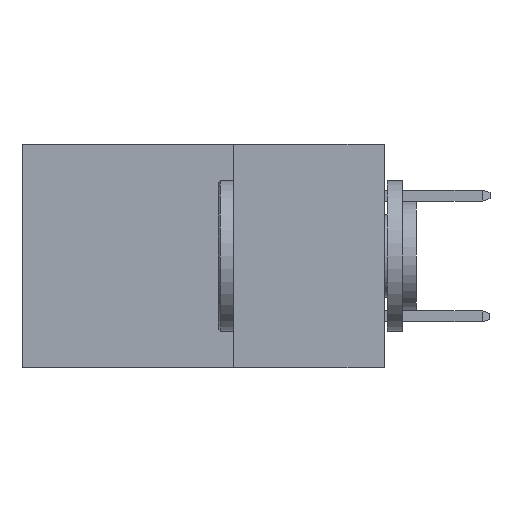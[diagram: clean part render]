
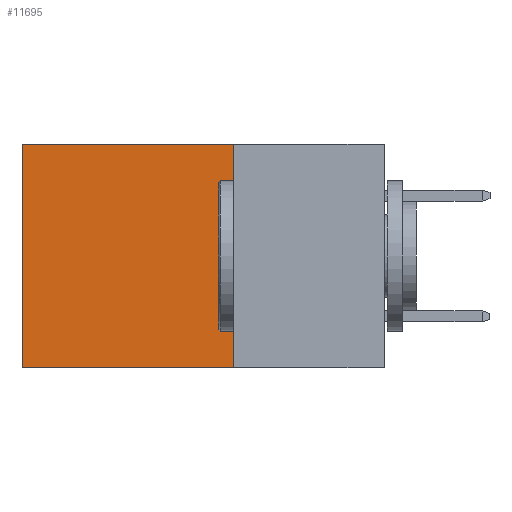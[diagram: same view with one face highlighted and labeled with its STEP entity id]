
A CAD part, left-side view. The second image highlights one B-rep face of the part: STEP entity #11695.
In plain terms, the highlighted planar face has unit normal (-1, 0, 0).
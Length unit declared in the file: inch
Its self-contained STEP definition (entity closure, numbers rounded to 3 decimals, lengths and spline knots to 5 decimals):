
#1762 = CARTESIAN_POINT ( 'NONE',  ( 0.298, 0.25, -0.37 ) ) ;
#3369 = AXIS2_PLACEMENT_3D ( 'NONE', #10174, #11344, #4335 ) ;
#3445 = LINE ( 'NONE', #13287, #9369 ) ;
#3631 = VERTEX_POINT ( 'NONE', #9866 ) ;
#4335 = DIRECTION ( 'NONE',  ( 0., 0., -1. ) ) ;
#4357 = CARTESIAN_POINT ( 'NONE',  ( 0.298, 0.25, 0. ) ) ;
#4647 = CARTESIAN_POINT ( 'NONE',  ( 0.298, 0.25, 0. ) ) ;
#4777 = CARTESIAN_POINT ( 'NONE',  ( 0.298, 0.25, -0.37 ) ) ;
#4915 = VERTEX_POINT ( 'NONE', #11802 ) ;
#5357 = CARTESIAN_POINT ( 'NONE',  ( 0.298, 0.6, 0. ) ) ;
#5767 = EDGE_CURVE ( 'NONE', #6051, #3631, #13843, .T. ) ;
#6051 = VERTEX_POINT ( 'NONE', #4647 ) ;
#7215 = ORIENTED_EDGE ( 'NONE', *, *, #11619, .T. ) ;
#7419 = ORIENTED_EDGE ( 'NONE', *, *, #12192, .F. ) ;
#7812 = PLANE ( 'NONE',  #3369 ) ;
#7878 = VECTOR ( 'NONE', #8910, 39.37008 ) ;
#8002 = VERTEX_POINT ( 'NONE', #1762 ) ;
#8353 = VECTOR ( 'NONE', #15155, 39.37008 ) ;
#8500 = ORIENTED_EDGE ( 'NONE', *, *, #9016, .F. ) ;
#8611 = EDGE_LOOP ( 'NONE', ( #7215, #8500, #7419, #14682 ) ) ;
#8910 = DIRECTION ( 'NONE',  ( 0., 0., -1. ) ) ;
#9016 = EDGE_CURVE ( 'NONE', #8002, #4915, #11465, .T. ) ;
#9369 = VECTOR ( 'NONE', #11075, 39.37008 ) ;
#9866 = CARTESIAN_POINT ( 'NONE',  ( 0.298, 0.6, 0. ) ) ;
#10174 = CARTESIAN_POINT ( 'NONE',  ( 0.298, 0.25, 0. ) ) ;
#10827 = VECTOR ( 'NONE', #12020, 39.37008 ) ;
#11075 = DIRECTION ( 'NONE',  ( 0., 0., -1. ) ) ;
#11344 = DIRECTION ( 'NONE',  ( 1., 0., 0. ) ) ;
#11465 = LINE ( 'NONE', #4777, #8353 ) ;
#11619 = EDGE_CURVE ( 'NONE', #3631, #4915, #14359, .T. ) ;
#11695 = ADVANCED_FACE ( 'NONE', ( #12943 ), #7812, .F. ) ;
#11802 = CARTESIAN_POINT ( 'NONE',  ( 0.298, 0.6, -0.37 ) ) ;
#12020 = DIRECTION ( 'NONE',  ( 0., 1., 0. ) ) ;
#12192 = EDGE_CURVE ( 'NONE', #6051, #8002, #3445, .T. ) ;
#12943 = FACE_OUTER_BOUND ( 'NONE', #8611, .T. ) ;
#13287 = CARTESIAN_POINT ( 'NONE',  ( 0.298, 0.25, 0. ) ) ;
#13843 = LINE ( 'NONE', #4357, #10827 ) ;
#14359 = LINE ( 'NONE', #5357, #7878 ) ;
#14682 = ORIENTED_EDGE ( 'NONE', *, *, #5767, .T. ) ;
#15155 = DIRECTION ( 'NONE',  ( 0., 1., 0. ) ) ;
